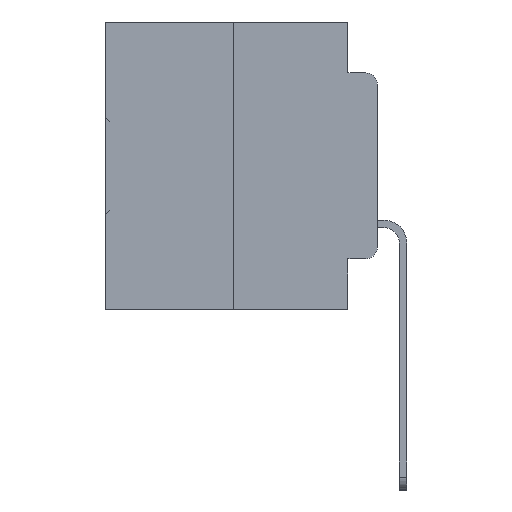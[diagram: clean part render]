
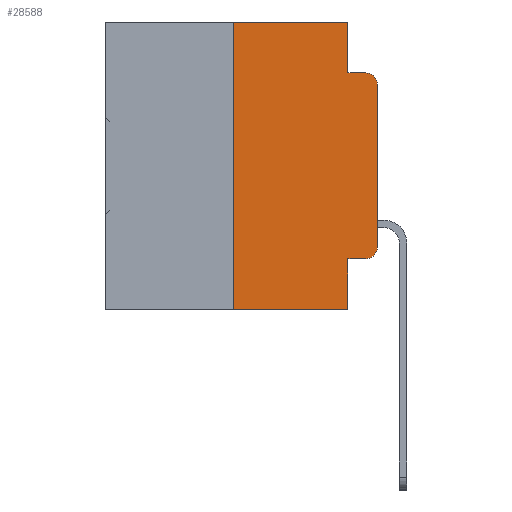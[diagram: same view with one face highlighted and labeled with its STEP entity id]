
A CAD part, left-side view. The second image highlights one B-rep face of the part: STEP entity #28588.
In plain terms, the highlighted planar face has unit normal (-1, 0, 0).
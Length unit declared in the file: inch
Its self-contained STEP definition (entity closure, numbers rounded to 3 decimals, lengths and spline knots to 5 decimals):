
#133 = VERTEX_POINT ( 'NONE', #22950 ) ;
#443 = CIRCLE ( 'NONE', #1023, 0.02 ) ;
#602 = AXIS2_PLACEMENT_3D ( 'NONE', #11435, #29718, #14081 ) ;
#1023 = AXIS2_PLACEMENT_3D ( 'NONE', #19354, #3575, #21976 ) ;
#2389 = CARTESIAN_POINT ( 'NONE',  ( 0., 0.02, -0.4115 ) ) ;
#2744 = CARTESIAN_POINT ( 'NONE',  ( 0., 0.25, -0.5 ) ) ;
#3552 = CARTESIAN_POINT ( 'NONE',  ( 0., 0.473, 0. ) ) ;
#3575 = DIRECTION ( 'NONE',  ( -1., 0., 0. ) ) ;
#3582 = DIRECTION ( 'NONE',  ( 0., 0., 1. ) ) ;
#4335 = VERTEX_POINT ( 'NONE', #2744 ) ;
#4418 = CARTESIAN_POINT ( 'NONE',  ( 0., 0.051, 0. ) ) ;
#4503 = VECTOR ( 'NONE', #19386, 39.37008 ) ;
#4770 = VERTEX_POINT ( 'NONE', #33410 ) ;
#4931 = VERTEX_POINT ( 'NONE', #23737 ) ;
#5328 = EDGE_CURVE ( 'NONE', #31691, #4931, #18790, .T. ) ;
#5442 = VERTEX_POINT ( 'NONE', #18102 ) ;
#6059 = EDGE_CURVE ( 'NONE', #11950, #23525, #16711, .T. ) ;
#6195 = DIRECTION ( 'NONE',  ( 1., 0., 0. ) ) ;
#6546 = LINE ( 'NONE', #32256, #33462 ) ;
#6565 = CARTESIAN_POINT ( 'NONE',  ( 0., 0.473, -0.5 ) ) ;
#11272 = EDGE_CURVE ( 'NONE', #133, #31691, #14868, .T. ) ;
#11435 = CARTESIAN_POINT ( 'NONE',  ( 0., 0.02, -0.3915 ) ) ;
#11904 = EDGE_LOOP ( 'NONE', ( #18420, #13070, #28596, #17228, #19670, #14327, #15151, #15987, #17633, #26214 ) ) ;
#11950 = VERTEX_POINT ( 'NONE', #23860 ) ;
#12928 = VECTOR ( 'NONE', #17200, 39.37008 ) ;
#13070 = ORIENTED_EDGE ( 'NONE', *, *, #18635, .T. ) ;
#14081 = DIRECTION ( 'NONE',  ( 0., 0., -1. ) ) ;
#14327 = ORIENTED_EDGE ( 'NONE', *, *, #19892, .F. ) ;
#14868 = LINE ( 'NONE', #23320, #27958 ) ;
#15057 = DIRECTION ( 'NONE',  ( 0., -1., 0. ) ) ;
#15151 = ORIENTED_EDGE ( 'NONE', *, *, #30965, .T. ) ;
#15907 = AXIS2_PLACEMENT_3D ( 'NONE', #3552, #6195, #24600 ) ;
#15987 = ORIENTED_EDGE ( 'NONE', *, *, #6059, .F. ) ;
#16711 = LINE ( 'NONE', #28108, #22822 ) ;
#16781 = CARTESIAN_POINT ( 'NONE',  ( 0., 0.25, 0. ) ) ;
#17111 = EDGE_CURVE ( 'NONE', #11950, #24864, #28137, .T. ) ;
#17200 = DIRECTION ( 'NONE',  ( 0., -1., 0. ) ) ;
#17228 = ORIENTED_EDGE ( 'NONE', *, *, #5328, .F. ) ;
#17633 = ORIENTED_EDGE ( 'NONE', *, *, #17111, .T. ) ;
#18085 = CARTESIAN_POINT ( 'NONE',  ( 0., 0.051, -0.5 ) ) ;
#18102 = CARTESIAN_POINT ( 'NONE',  ( 0., 0., -0.1085 ) ) ;
#18420 = ORIENTED_EDGE ( 'NONE', *, *, #20397, .T. ) ;
#18635 = EDGE_CURVE ( 'NONE', #5442, #19463, #443, .T. ) ;
#18790 = LINE ( 'NONE', #25448, #30956 ) ;
#19354 = CARTESIAN_POINT ( 'NONE',  ( 0., 0.02, -0.1085 ) ) ;
#19386 = DIRECTION ( 'NONE',  ( 0., 0., 1. ) ) ;
#19463 = VERTEX_POINT ( 'NONE', #25273 ) ;
#19670 = ORIENTED_EDGE ( 'NONE', *, *, #11272, .F. ) ;
#19892 = EDGE_CURVE ( 'NONE', #4335, #133, #31503, .T. ) ;
#19912 = LINE ( 'NONE', #6565, #12928 ) ;
#20379 = EDGE_CURVE ( 'NONE', #24864, #4770, #28296, .T. ) ;
#20397 = EDGE_CURVE ( 'NONE', #4770, #5442, #6546, .T. ) ;
#21976 = DIRECTION ( 'NONE',  ( 0., 0., -1. ) ) ;
#22349 = FACE_OUTER_BOUND ( 'NONE', #11904, .T. ) ;
#22822 = VECTOR ( 'NONE', #25621, 39.37008 ) ;
#22904 = CARTESIAN_POINT ( 'NONE',  ( 0., 0.051, -0.0885 ) ) ;
#22950 = CARTESIAN_POINT ( 'NONE',  ( 0., 0.25, 0. ) ) ;
#23320 = CARTESIAN_POINT ( 'NONE',  ( 0., 0.473, 0. ) ) ;
#23525 = VERTEX_POINT ( 'NONE', #18085 ) ;
#23657 = VECTOR ( 'NONE', #15057, 39.37008 ) ;
#23737 = CARTESIAN_POINT ( 'NONE',  ( 0., 0.051, -0.0885 ) ) ;
#23860 = CARTESIAN_POINT ( 'NONE',  ( 0., 0.051, -0.4115 ) ) ;
#24483 = PLANE ( 'NONE',  #15907 ) ;
#24600 = DIRECTION ( 'NONE',  ( 0., 0., -1. ) ) ;
#24864 = VERTEX_POINT ( 'NONE', #2389 ) ;
#25273 = CARTESIAN_POINT ( 'NONE',  ( 0., 0.02, -0.0885 ) ) ;
#25448 = CARTESIAN_POINT ( 'NONE',  ( 0., 0.051, 0. ) ) ;
#25553 = DIRECTION ( 'NONE',  ( 0., -1., 0. ) ) ;
#25621 = DIRECTION ( 'NONE',  ( 0., 0., -1. ) ) ;
#25790 = VECTOR ( 'NONE', #25553, 39.37008 ) ;
#25957 = DIRECTION ( 'NONE',  ( 0., -1., 0. ) ) ;
#26214 = ORIENTED_EDGE ( 'NONE', *, *, #20379, .T. ) ;
#26601 = LINE ( 'NONE', #22904, #25790 ) ;
#27958 = VECTOR ( 'NONE', #25957, 39.37008 ) ;
#28038 = DIRECTION ( 'NONE',  ( 0., 0., -1. ) ) ;
#28108 = CARTESIAN_POINT ( 'NONE',  ( 0., 0.051, 0. ) ) ;
#28137 = LINE ( 'NONE', #30656, #23657 ) ;
#28296 = CIRCLE ( 'NONE', #602, 0.02 ) ;
#28588 = ADVANCED_FACE ( 'NONE', ( #22349 ), #24483, .F. ) ;
#28596 = ORIENTED_EDGE ( 'NONE', *, *, #33625, .F. ) ;
#29718 = DIRECTION ( 'NONE',  ( -1., 0., 0. ) ) ;
#30656 = CARTESIAN_POINT ( 'NONE',  ( 0., 0.051, -0.4115 ) ) ;
#30956 = VECTOR ( 'NONE', #28038, 39.37008 ) ;
#30965 = EDGE_CURVE ( 'NONE', #4335, #23525, #19912, .T. ) ;
#31503 = LINE ( 'NONE', #16781, #4503 ) ;
#31691 = VERTEX_POINT ( 'NONE', #4418 ) ;
#32256 = CARTESIAN_POINT ( 'NONE',  ( 0., 0., 0. ) ) ;
#33410 = CARTESIAN_POINT ( 'NONE',  ( 0., 0., -0.3915 ) ) ;
#33462 = VECTOR ( 'NONE', #3582, 39.37008 ) ;
#33625 = EDGE_CURVE ( 'NONE', #4931, #19463, #26601, .T. ) ;
